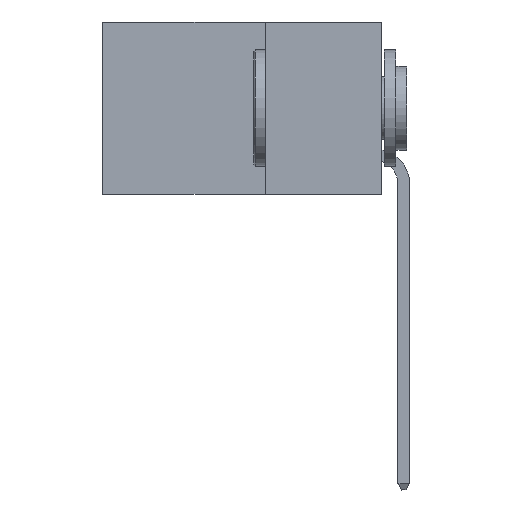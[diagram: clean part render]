
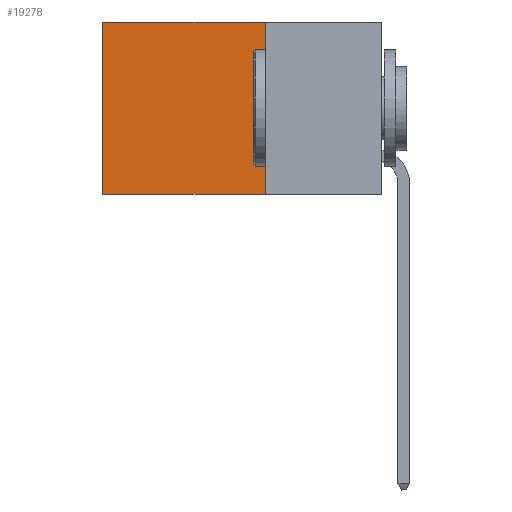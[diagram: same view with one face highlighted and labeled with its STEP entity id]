
A CAD part, left-side view. The second image highlights one B-rep face of the part: STEP entity #19278.
In plain terms, the highlighted planar face has unit normal (-1, 0, 0).
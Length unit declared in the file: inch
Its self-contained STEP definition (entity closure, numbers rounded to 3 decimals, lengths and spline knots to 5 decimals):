
#678 = VECTOR ( 'NONE', #13138, 39.37008 ) ;
#1505 = EDGE_CURVE ( 'NONE', #6117, #23211, #21269, .T. ) ;
#2370 = VECTOR ( 'NONE', #11358, 39.37008 ) ;
#3266 = FACE_OUTER_BOUND ( 'NONE', #4892, .T. ) ;
#3424 = ORIENTED_EDGE ( 'NONE', *, *, #27927, .F. ) ;
#3978 = EDGE_CURVE ( 'NONE', #6117, #28747, #4509, .T. ) ;
#4509 = LINE ( 'NONE', #17781, #678 ) ;
#4892 = EDGE_LOOP ( 'NONE', ( #11006, #3424, #14740, #23269 ) ) ;
#6079 = DIRECTION ( 'NONE',  ( 0., 1., 0. ) ) ;
#6117 = VERTEX_POINT ( 'NONE', #17848 ) ;
#7871 = CARTESIAN_POINT ( 'NONE',  ( 0.2875, 0.25, -0.37 ) ) ;
#8558 = VERTEX_POINT ( 'NONE', #27651 ) ;
#9096 = LINE ( 'NONE', #13930, #2370 ) ;
#10980 = DIRECTION ( 'NONE',  ( 0., 0., -1. ) ) ;
#11006 = ORIENTED_EDGE ( 'NONE', *, *, #29144, .T. ) ;
#11279 = DIRECTION ( 'NONE',  ( 1., 0., 0. ) ) ;
#11358 = DIRECTION ( 'NONE',  ( 0., 0., -1. ) ) ;
#11869 = CARTESIAN_POINT ( 'NONE',  ( 0.2875, 0.6, 0. ) ) ;
#12866 = PLANE ( 'NONE',  #21872 ) ;
#12954 = CARTESIAN_POINT ( 'NONE',  ( 0.2875, 0.25, -0.37 ) ) ;
#13138 = DIRECTION ( 'NONE',  ( 0., 0., -1. ) ) ;
#13930 = CARTESIAN_POINT ( 'NONE',  ( 0.2875, 0.6, 0. ) ) ;
#14740 = ORIENTED_EDGE ( 'NONE', *, *, #3978, .F. ) ;
#17420 = CARTESIAN_POINT ( 'NONE',  ( 0.2875, 0.25, 0. ) ) ;
#17781 = CARTESIAN_POINT ( 'NONE',  ( 0.2875, 0.25, 0. ) ) ;
#17848 = CARTESIAN_POINT ( 'NONE',  ( 0.2875, 0.25, 0. ) ) ;
#19278 = ADVANCED_FACE ( 'NONE', ( #3266 ), #12866, .F. ) ;
#19608 = DIRECTION ( 'NONE',  ( 0., 1., 0. ) ) ;
#19787 = VECTOR ( 'NONE', #6079, 39.37008 ) ;
#21269 = LINE ( 'NONE', #21968, #21600 ) ;
#21600 = VECTOR ( 'NONE', #19608, 39.37008 ) ;
#21872 = AXIS2_PLACEMENT_3D ( 'NONE', #17420, #11279, #10980 ) ;
#21968 = CARTESIAN_POINT ( 'NONE',  ( 0.2875, 0.25, 0. ) ) ;
#23211 = VERTEX_POINT ( 'NONE', #11869 ) ;
#23269 = ORIENTED_EDGE ( 'NONE', *, *, #1505, .T. ) ;
#23684 = LINE ( 'NONE', #12954, #19787 ) ;
#27651 = CARTESIAN_POINT ( 'NONE',  ( 0.2875, 0.6, -0.37 ) ) ;
#27927 = EDGE_CURVE ( 'NONE', #28747, #8558, #23684, .T. ) ;
#28747 = VERTEX_POINT ( 'NONE', #7871 ) ;
#29144 = EDGE_CURVE ( 'NONE', #23211, #8558, #9096, .T. ) ;
